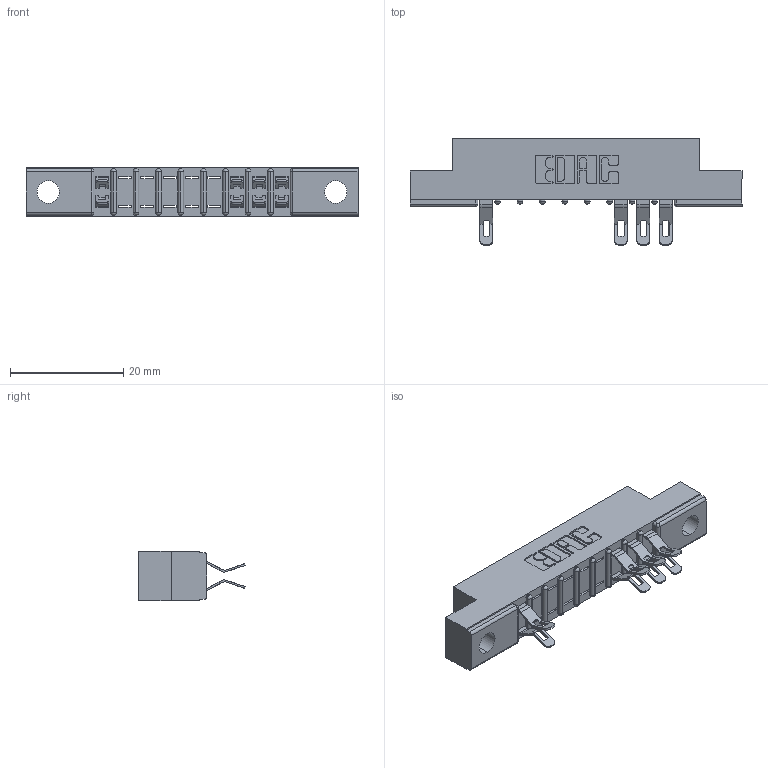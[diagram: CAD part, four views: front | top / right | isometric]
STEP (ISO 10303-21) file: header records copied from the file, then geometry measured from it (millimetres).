
FILE_DESCRIPTION (( 'STEP AP203' ), '1' );
FILE_NAME ('357-018-555-204.STEP', '2018-08-08T05:42:42', ( '' ), ( '' ), 'SwSTEP 2.0', 'SolidWorks 2016', '' );
FILE_SCHEMA (( 'CONFIG_CONTROL_DESIGN' ));
Length unit declared in the file: inch
Products named in the file (3): 307 Part_.156 Dia Mounting Holes; 307-290-001_555; 357-018-555-204
Assembly tree (9 placements, depth 2):
  357-018-555-204
    307 Part_.156 Dia Mounting Holes
    307-290-001_555  x8
Bounding box: 58.67 x 18.75 x 8.71 mm (x, y, z)
Volume: 3627.8 mm3; surface area: 4985.1 mm2
Topology: 9 solids, 9 shells, 730 faces, 2127 edges, 1378 vertices
Faces by surface type: plane 416, cylinder 294, sphere 20
Entity records: 12707 total; most frequent: CARTESIAN_POINT 2141, ORIENTED_EDGE 2128, DIRECTION 2100, EDGE_CURVE 1064, VECTOR 798, LINE 798, VERTEX_POINT 692, AXIS2_PLACEMENT_3D 651
